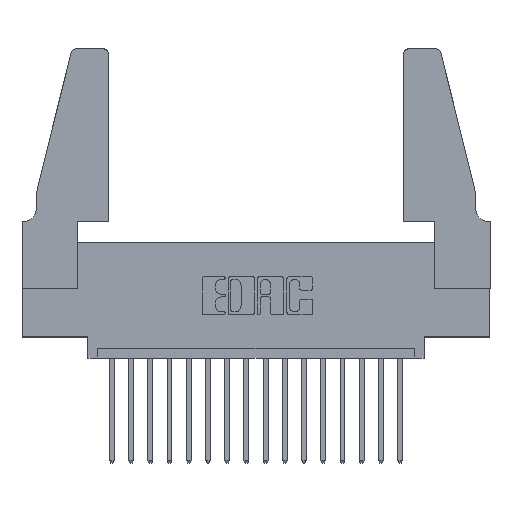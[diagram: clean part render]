
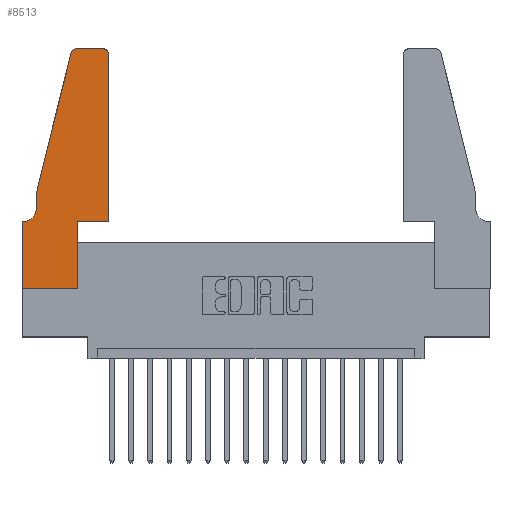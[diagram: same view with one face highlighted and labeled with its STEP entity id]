
A CAD part, top view. The second image highlights one B-rep face of the part: STEP entity #8513.
In plain terms, the highlighted planar face has unit normal (0, 0, 1).
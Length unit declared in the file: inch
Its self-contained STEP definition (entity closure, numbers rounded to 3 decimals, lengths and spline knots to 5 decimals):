
#29 = DIRECTION ( 'NONE',  ( 1., 0., 0. ) ) ;
#236 = VERTEX_POINT ( 'NONE', #1599 ) ;
#241 = ORIENTED_EDGE ( 'NONE', *, *, #16532, .T. ) ;
#782 = EDGE_CURVE ( 'NONE', #5874, #5997, #1439, .T. ) ;
#801 = ORIENTED_EDGE ( 'NONE', *, *, #782, .T. ) ;
#821 = DIRECTION ( 'NONE',  ( -1., 0., 0. ) ) ;
#898 = CARTESIAN_POINT ( 'NONE',  ( 0.4505, 0.35, 0.37 ) ) ;
#1079 = CARTESIAN_POINT ( 'NONE',  ( 0.0755, 0.5, 0.37 ) ) ;
#1299 = AXIS2_PLACEMENT_3D ( 'NONE', #14886, #13588, #5159 ) ;
#1334 = CARTESIAN_POINT ( 'NONE',  ( 0.4505, 0.35, 0.37 ) ) ;
#1439 = LINE ( 'NONE', #13631, #9939 ) ;
#1460 = VECTOR ( 'NONE', #10759, 39.37008 ) ;
#1554 = EDGE_CURVE ( 'NONE', #2577, #14396, #15720, .T. ) ;
#1599 = CARTESIAN_POINT ( 'NONE',  ( 0.4205, 1.25, 0.37 ) ) ;
#2159 = EDGE_CURVE ( 'NONE', #15742, #11818, #6010, .T. ) ;
#2242 = DIRECTION ( 'NONE',  ( 0., 1., 0. ) ) ;
#2368 = ORIENTED_EDGE ( 'NONE', *, *, #16828, .T. ) ;
#2370 = CARTESIAN_POINT ( 'NONE',  ( 0.0755, 0.5, 0.37 ) ) ;
#2577 = VERTEX_POINT ( 'NONE', #1079 ) ;
#2657 = VERTEX_POINT ( 'NONE', #3816 ) ;
#3409 = DIRECTION ( 'NONE',  ( 1., 0., 0. ) ) ;
#3595 = VECTOR ( 'NONE', #29, 39.37008 ) ;
#3763 = CIRCLE ( 'NONE', #16582, 0.07 ) ;
#3816 = CARTESIAN_POINT ( 'NONE',  ( 0., 0., 0.37 ) ) ;
#3912 = DIRECTION ( 'NONE',  ( -1., 0., 0. ) ) ;
#3938 = VECTOR ( 'NONE', #8130, 39.37008 ) ;
#4035 = DIRECTION ( 'NONE',  ( 0., 1., 0. ) ) ;
#4057 = AXIS2_PLACEMENT_3D ( 'NONE', #6189, #16084, #7828 ) ;
#4083 = LINE ( 'NONE', #898, #9310 ) ;
#4397 = EDGE_CURVE ( 'NONE', #2657, #5874, #8956, .T. ) ;
#4545 = ORIENTED_EDGE ( 'NONE', *, *, #4397, .T. ) ;
#4620 = DIRECTION ( 'NONE',  ( 0., 0., 1. ) ) ;
#4636 = VERTEX_POINT ( 'NONE', #15310 ) ;
#4685 = VECTOR ( 'NONE', #17604, 39.37008 ) ;
#5159 = DIRECTION ( 'NONE',  ( 1., 0., 0. ) ) ;
#5224 = PLANE ( 'NONE',  #1299 ) ;
#5328 = CARTESIAN_POINT ( 'NONE',  ( 0., 0., 0.37 ) ) ;
#5401 = CIRCLE ( 'NONE', #6842, 0.03 ) ;
#5874 = VERTEX_POINT ( 'NONE', #16758 ) ;
#5997 = VERTEX_POINT ( 'NONE', #11503 ) ;
#6010 = LINE ( 'NONE', #6917, #4685 ) ;
#6053 = CARTESIAN_POINT ( 'NONE',  ( 0.4505, 1.22, 0.37 ) ) ;
#6189 = CARTESIAN_POINT ( 'NONE',  ( 0.4205, 1.22, 0.37 ) ) ;
#6282 = LINE ( 'NONE', #10675, #8467 ) ;
#6567 = DIRECTION ( 'NONE',  ( 0., -1., 0. ) ) ;
#6842 = AXIS2_PLACEMENT_3D ( 'NONE', #17171, #4620, #3409 ) ;
#6917 = CARTESIAN_POINT ( 'NONE',  ( 0.0755, 0.35, 0.37 ) ) ;
#7113 = ORIENTED_EDGE ( 'NONE', *, *, #15224, .T. ) ;
#7308 = LINE ( 'NONE', #1334, #3595 ) ;
#7732 = DIRECTION ( 'NONE',  ( 0., 0., -1. ) ) ;
#7828 = DIRECTION ( 'NONE',  ( 1., 0., 0. ) ) ;
#7938 = ORIENTED_EDGE ( 'NONE', *, *, #15997, .T. ) ;
#8100 = EDGE_CURVE ( 'NONE', #14396, #15742, #3763, .T. ) ;
#8130 = DIRECTION ( 'NONE',  ( 1., 0., 0. ) ) ;
#8467 = VECTOR ( 'NONE', #6567, 39.37008 ) ;
#8480 = ORIENTED_EDGE ( 'NONE', *, *, #14627, .T. ) ;
#8513 = ADVANCED_FACE ( 'NONE', ( #10066 ), #5224, .T. ) ;
#8956 = LINE ( 'NONE', #5328, #3938 ) ;
#9268 = LINE ( 'NONE', #11062, #13101 ) ;
#9310 = VECTOR ( 'NONE', #2242, 39.37008 ) ;
#9627 = CARTESIAN_POINT ( 'NONE',  ( 0.0755, 0.42, 0.37 ) ) ;
#9939 = VECTOR ( 'NONE', #4035, 39.37008 ) ;
#10066 = FACE_OUTER_BOUND ( 'NONE', #15053, .T. ) ;
#10675 = CARTESIAN_POINT ( 'NONE',  ( 0., 0., 0.37 ) ) ;
#10759 = DIRECTION ( 'NONE',  ( 0., -1., 0. ) ) ;
#11062 = CARTESIAN_POINT ( 'NONE',  ( 0.0755, 0.5, 0.37 ) ) ;
#11503 = CARTESIAN_POINT ( 'NONE',  ( 0.2865, 0.35, 0.37 ) ) ;
#11818 = VERTEX_POINT ( 'NONE', #14569 ) ;
#12054 = VERTEX_POINT ( 'NONE', #16819 ) ;
#12212 = ORIENTED_EDGE ( 'NONE', *, *, #1554, .T. ) ;
#12268 = CARTESIAN_POINT ( 'NONE',  ( 0.4505, 0.35, 0.37 ) ) ;
#12440 = CIRCLE ( 'NONE', #4057, 0.03 ) ;
#12794 = VERTEX_POINT ( 'NONE', #12268 ) ;
#13101 = VECTOR ( 'NONE', #14048, 39.37008 ) ;
#13527 = CARTESIAN_POINT ( 'NONE',  ( 0.0055, 0.35, 0.37 ) ) ;
#13588 = DIRECTION ( 'NONE',  ( 0., 0., 1. ) ) ;
#13631 = CARTESIAN_POINT ( 'NONE',  ( 0.2865, 0.35, 0.37 ) ) ;
#13815 = LINE ( 'NONE', #15102, #14897 ) ;
#14048 = DIRECTION ( 'NONE',  ( -0.239, -0.971, 0. ) ) ;
#14396 = VERTEX_POINT ( 'NONE', #9627 ) ;
#14569 = CARTESIAN_POINT ( 'NONE',  ( 0., 0.35, 0.37 ) ) ;
#14627 = EDGE_CURVE ( 'NONE', #4636, #12054, #5401, .T. ) ;
#14886 = CARTESIAN_POINT ( 'NONE',  ( 0., 0.35, 0.37 ) ) ;
#14897 = VECTOR ( 'NONE', #3912, 39.37008 ) ;
#14931 = EDGE_CURVE ( 'NONE', #11818, #2657, #6282, .T. ) ;
#15053 = EDGE_LOOP ( 'NONE', ( #7113, #8480, #7938, #12212, #16741, #17150, #16238, #4545, #801, #241, #17810, #2368 ) ) ;
#15089 = EDGE_CURVE ( 'NONE', #12794, #17323, #4083, .T. ) ;
#15102 = CARTESIAN_POINT ( 'NONE',  ( 0.2605, 1.25, 0.37 ) ) ;
#15224 = EDGE_CURVE ( 'NONE', #236, #4636, #13815, .T. ) ;
#15310 = CARTESIAN_POINT ( 'NONE',  ( 0.284, 1.25, 0.37 ) ) ;
#15720 = LINE ( 'NONE', #2370, #1460 ) ;
#15742 = VERTEX_POINT ( 'NONE', #13527 ) ;
#15997 = EDGE_CURVE ( 'NONE', #12054, #2577, #9268, .T. ) ;
#16003 = CARTESIAN_POINT ( 'NONE',  ( 0.0055, 0.42, 0.37 ) ) ;
#16084 = DIRECTION ( 'NONE',  ( 0., 0., 1. ) ) ;
#16238 = ORIENTED_EDGE ( 'NONE', *, *, #14931, .T. ) ;
#16532 = EDGE_CURVE ( 'NONE', #5997, #12794, #7308, .T. ) ;
#16582 = AXIS2_PLACEMENT_3D ( 'NONE', #16003, #7732, #821 ) ;
#16741 = ORIENTED_EDGE ( 'NONE', *, *, #8100, .T. ) ;
#16758 = CARTESIAN_POINT ( 'NONE',  ( 0.2865, 0., 0.37 ) ) ;
#16819 = CARTESIAN_POINT ( 'NONE',  ( 0.25487, 1.22718, 0.37 ) ) ;
#16828 = EDGE_CURVE ( 'NONE', #17323, #236, #12440, .T. ) ;
#17150 = ORIENTED_EDGE ( 'NONE', *, *, #2159, .T. ) ;
#17171 = CARTESIAN_POINT ( 'NONE',  ( 0.284, 1.22, 0.37 ) ) ;
#17323 = VERTEX_POINT ( 'NONE', #6053 ) ;
#17604 = DIRECTION ( 'NONE',  ( -1., 0., 0. ) ) ;
#17810 = ORIENTED_EDGE ( 'NONE', *, *, #15089, .T. ) ;
